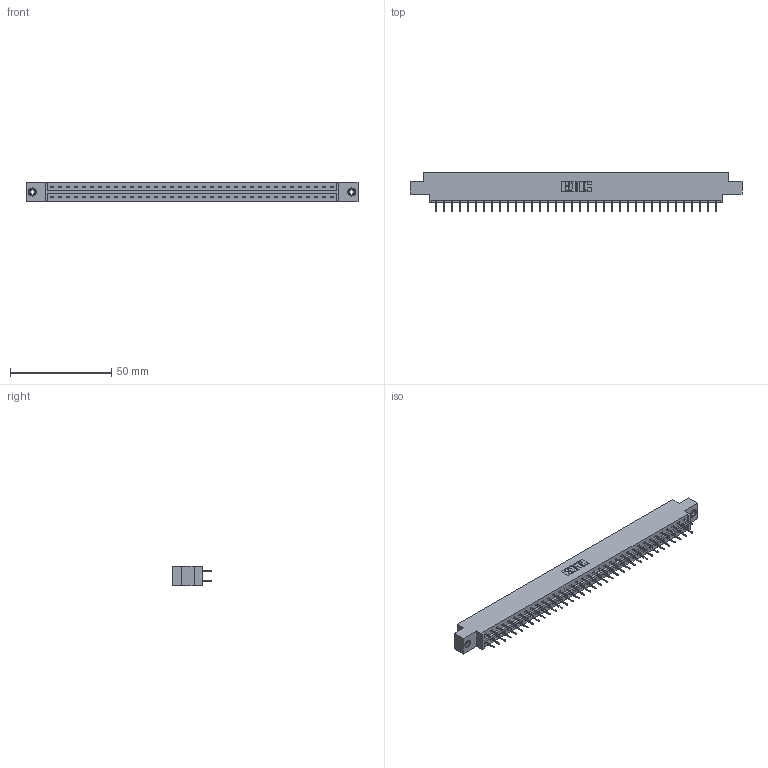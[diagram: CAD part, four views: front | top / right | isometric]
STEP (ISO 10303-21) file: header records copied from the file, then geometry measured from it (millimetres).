
FILE_DESCRIPTION (( 'STEP AP203' ), '1' );
FILE_NAME ('833-072-524-808.STEP', '2020-06-05T14:07:57', ( '' ), ( '' ), 'SwSTEP 2.0', 'SolidWorks 2020', '' );
FILE_SCHEMA (( 'CONFIG_CONTROL_DESIGN' ));
Length unit declared in the file: inch
Products named in the file (4): 833 Part_Offset - .156 Dia - TI; 833-072-524-808; 345-250-001_345-250-003-102; 345-292-001_345-293-124
Assembly tree (75 placements, depth 2):
  833-072-524-808
    833 Part_Offset - .156 Dia - TI
    345-292-001_345-293-124  x72
    345-250-001_345-250-003-102  x2
Bounding box: 164.19 x 19.69 x 9.4 mm (x, y, z)
Volume: 16363 mm3; surface area: 19196.3 mm2
Topology: 75 solids, 75 shells, 4210 faces, 11907 edges, 7642 vertices
Faces by surface type: plane 3130, cylinder 1064, cone 12, torus 4
Entity records: 25328 total; most frequent: CARTESIAN_POINT 4189, ORIENTED_EDGE 4118, DIRECTION 3621, EDGE_CURVE 2059, LINE 1915, VECTOR 1915, VERTEX_POINT 1364, AXIS2_PLACEMENT_3D 853
